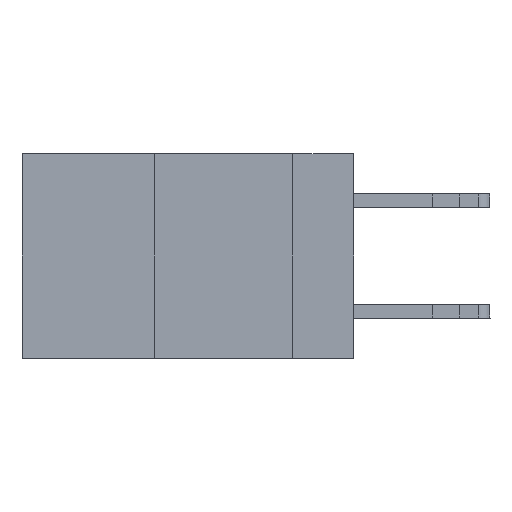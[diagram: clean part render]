
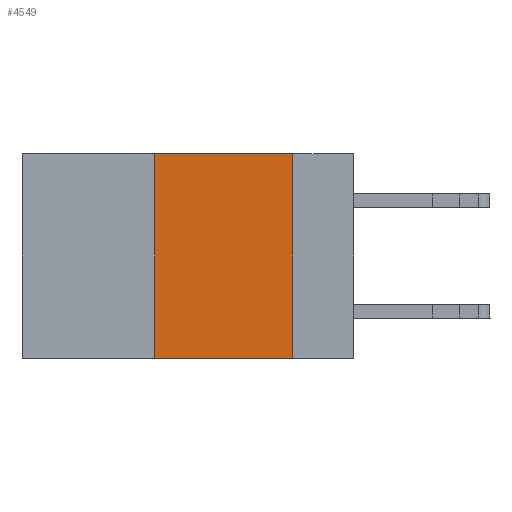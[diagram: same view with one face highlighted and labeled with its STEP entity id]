
A CAD part, left-side view. The second image highlights one B-rep face of the part: STEP entity #4549.
In plain terms, the highlighted planar face has unit normal (-1, 0, 0).
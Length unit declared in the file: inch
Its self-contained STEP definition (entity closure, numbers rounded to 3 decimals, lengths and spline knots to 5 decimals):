
#45 = VECTOR ( 'NONE', #20938, 39.37008 ) ;
#488 = LINE ( 'NONE', #15833, #45 ) ;
#2143 = VERTEX_POINT ( 'NONE', #11456 ) ;
#3139 = DIRECTION ( 'NONE',  ( 0., 0., -1. ) ) ;
#3923 = CARTESIAN_POINT ( 'NONE',  ( 0., 0.36, 0. ) ) ;
#4454 = EDGE_CURVE ( 'NONE', #7295, #8663, #10660, .T. ) ;
#4549 = ADVANCED_FACE ( 'NONE', ( #16432 ), #6438, .F. ) ;
#4833 = CARTESIAN_POINT ( 'NONE',  ( 0., 0.11, 0. ) ) ;
#6438 = PLANE ( 'NONE',  #16642 ) ;
#6753 = DIRECTION ( 'NONE',  ( 1., 0., 0. ) ) ;
#7203 = CARTESIAN_POINT ( 'NONE',  ( 0., 0.11, 0. ) ) ;
#7295 = VERTEX_POINT ( 'NONE', #17254 ) ;
#7342 = CARTESIAN_POINT ( 'NONE',  ( 0., 0.6, 0. ) ) ;
#8128 = ORIENTED_EDGE ( 'NONE', *, *, #4454, .F. ) ;
#8663 = VERTEX_POINT ( 'NONE', #7203 ) ;
#9210 = EDGE_CURVE ( 'NONE', #2143, #13382, #488, .T. ) ;
#9786 = ORIENTED_EDGE ( 'NONE', *, *, #16439, .F. ) ;
#10596 = VECTOR ( 'NONE', #20870, 39.37008 ) ;
#10660 = LINE ( 'NONE', #7342, #10596 ) ;
#10691 = DIRECTION ( 'NONE',  ( 0., 0., 1. ) ) ;
#11456 = CARTESIAN_POINT ( 'NONE',  ( 0., 0.36, -0.37 ) ) ;
#11512 = ORIENTED_EDGE ( 'NONE', *, *, #9210, .T. ) ;
#11867 = CARTESIAN_POINT ( 'NONE',  ( 0., 0.6, 0. ) ) ;
#11942 = VECTOR ( 'NONE', #3139, 39.37008 ) ;
#12968 = ORIENTED_EDGE ( 'NONE', *, *, #14048, .F. ) ;
#13382 = VERTEX_POINT ( 'NONE', #18520 ) ;
#14048 = EDGE_CURVE ( 'NONE', #2143, #7295, #21127, .T. ) ;
#14100 = EDGE_LOOP ( 'NONE', ( #9786, #8128, #12968, #11512 ) ) ;
#15005 = LINE ( 'NONE', #4833, #11942 ) ;
#15833 = CARTESIAN_POINT ( 'NONE',  ( 0., 0.6, -0.37 ) ) ;
#16432 = FACE_OUTER_BOUND ( 'NONE', #14100, .T. ) ;
#16439 = EDGE_CURVE ( 'NONE', #8663, #13382, #15005, .T. ) ;
#16642 = AXIS2_PLACEMENT_3D ( 'NONE', #11867, #6753, #18654 ) ;
#17254 = CARTESIAN_POINT ( 'NONE',  ( 0., 0.36, 0. ) ) ;
#18520 = CARTESIAN_POINT ( 'NONE',  ( 0., 0.11, -0.37 ) ) ;
#18654 = DIRECTION ( 'NONE',  ( 0., 0., -1. ) ) ;
#20870 = DIRECTION ( 'NONE',  ( 0., -1., 0. ) ) ;
#20938 = DIRECTION ( 'NONE',  ( 0., -1., 0. ) ) ;
#21127 = LINE ( 'NONE', #3923, #21454 ) ;
#21454 = VECTOR ( 'NONE', #10691, 39.37008 ) ;
